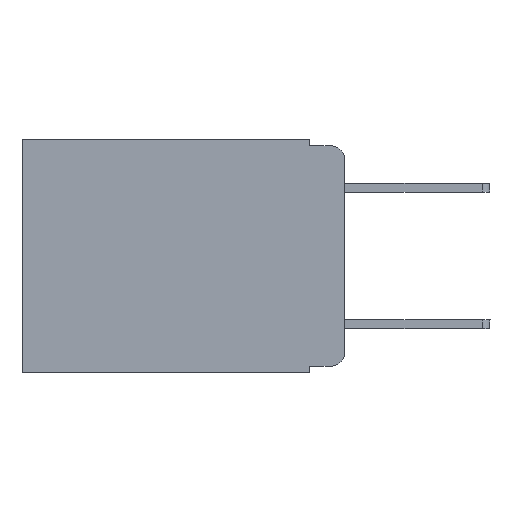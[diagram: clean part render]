
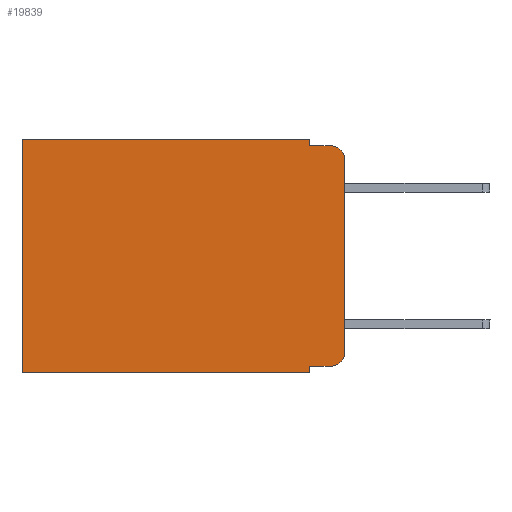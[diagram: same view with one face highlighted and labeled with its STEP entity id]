
A CAD part, left-side view. The second image highlights one B-rep face of the part: STEP entity #19839.
In plain terms, the highlighted planar face has unit normal (-1, 0, 0).
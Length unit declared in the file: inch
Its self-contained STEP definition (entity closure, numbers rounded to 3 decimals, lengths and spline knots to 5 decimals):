
#256 = CARTESIAN_POINT ( 'NONE',  ( 0.298, 0.051, 0. ) ) ;
#275 = VECTOR ( 'NONE', #21660, 39.37008 ) ;
#286 = ORIENTED_EDGE ( 'NONE', *, *, #16755, .T. ) ;
#448 = ORIENTED_EDGE ( 'NONE', *, *, #10956, .F. ) ;
#459 = CARTESIAN_POINT ( 'NONE',  ( 0.298, 0.02, -0.01 ) ) ;
#552 = CARTESIAN_POINT ( 'NONE',  ( 0.298, 0.051, -0.01 ) ) ;
#755 = AXIS2_PLACEMENT_3D ( 'NONE', #16500, #15062, #11660 ) ;
#1377 = EDGE_CURVE ( 'NONE', #11812, #21013, #11252, .T. ) ;
#1898 = FACE_OUTER_BOUND ( 'NONE', #20386, .T. ) ;
#2099 = ORIENTED_EDGE ( 'NONE', *, *, #1377, .F. ) ;
#2185 = LINE ( 'NONE', #2499, #13673 ) ;
#2336 = DIRECTION ( 'NONE',  ( -1., 0., 0. ) ) ;
#2499 = CARTESIAN_POINT ( 'NONE',  ( 0.298, 0.051, 0. ) ) ;
#2699 = CARTESIAN_POINT ( 'NONE',  ( 0.298, 0., 0. ) ) ;
#2823 = DIRECTION ( 'NONE',  ( 0., 1., 0. ) ) ;
#2833 = AXIS2_PLACEMENT_3D ( 'NONE', #18126, #3065, #6771 ) ;
#3065 = DIRECTION ( 'NONE',  ( -1., 0., 0. ) ) ;
#3127 = VERTEX_POINT ( 'NONE', #4134 ) ;
#3799 = VECTOR ( 'NONE', #15537, 39.37008 ) ;
#3920 = EDGE_CURVE ( 'NONE', #7084, #5187, #10862, .T. ) ;
#3995 = CARTESIAN_POINT ( 'NONE',  ( 0.298, 0., -0.313 ) ) ;
#4134 = CARTESIAN_POINT ( 'NONE',  ( 0.298, 0.473, 0. ) ) ;
#4541 = LINE ( 'NONE', #16174, #5563 ) ;
#5187 = VERTEX_POINT ( 'NONE', #459 ) ;
#5304 = CARTESIAN_POINT ( 'NONE',  ( 0.298, 0.02, -0.313 ) ) ;
#5563 = VECTOR ( 'NONE', #21149, 39.37008 ) ;
#5812 = ORIENTED_EDGE ( 'NONE', *, *, #6249, .T. ) ;
#6001 = ORIENTED_EDGE ( 'NONE', *, *, #7471, .F. ) ;
#6236 = VECTOR ( 'NONE', #14060, 39.37008 ) ;
#6249 = EDGE_CURVE ( 'NONE', #7982, #3127, #15973, .T. ) ;
#6476 = CARTESIAN_POINT ( 'NONE',  ( 0.298, 0., -0.343 ) ) ;
#6595 = VERTEX_POINT ( 'NONE', #17065 ) ;
#6627 = CARTESIAN_POINT ( 'NONE',  ( 0.298, 0.02, -0.333 ) ) ;
#6771 = DIRECTION ( 'NONE',  ( 0., 0., -1. ) ) ;
#6863 = ORIENTED_EDGE ( 'NONE', *, *, #15277, .F. ) ;
#7037 = CARTESIAN_POINT ( 'NONE',  ( 0.298, 0.051, -0.01 ) ) ;
#7084 = VERTEX_POINT ( 'NONE', #7037 ) ;
#7381 = DIRECTION ( 'NONE',  ( 0., 0., -1. ) ) ;
#7471 = EDGE_CURVE ( 'NONE', #6595, #19895, #2185, .T. ) ;
#7644 = VECTOR ( 'NONE', #17146, 39.37008 ) ;
#7768 = CARTESIAN_POINT ( 'NONE',  ( 0.298, 0., -0.03 ) ) ;
#7982 = VERTEX_POINT ( 'NONE', #19497 ) ;
#9092 = AXIS2_PLACEMENT_3D ( 'NONE', #5304, #2336, #7381 ) ;
#9336 = LINE ( 'NONE', #14266, #6236 ) ;
#9562 = LINE ( 'NONE', #6476, #275 ) ;
#10462 = LINE ( 'NONE', #256, #3799 ) ;
#10829 = ORIENTED_EDGE ( 'NONE', *, *, #3920, .F. ) ;
#10862 = LINE ( 'NONE', #552, #7644 ) ;
#10956 = EDGE_CURVE ( 'NONE', #7982, #7084, #10462, .T. ) ;
#11252 = LINE ( 'NONE', #2699, #15137 ) ;
#11360 = CARTESIAN_POINT ( 'NONE',  ( 0.298, 0., 0. ) ) ;
#11660 = DIRECTION ( 'NONE',  ( 0., 0., -1. ) ) ;
#11812 = VERTEX_POINT ( 'NONE', #7768 ) ;
#11882 = CIRCLE ( 'NONE', #9092, 0.02 ) ;
#12731 = EDGE_CURVE ( 'NONE', #11812, #5187, #20363, .T. ) ;
#13399 = PLANE ( 'NONE',  #755 ) ;
#13600 = CARTESIAN_POINT ( 'NONE',  ( 0.298, 0.051, -0.343 ) ) ;
#13673 = VECTOR ( 'NONE', #17553, 39.37008 ) ;
#13767 = ORIENTED_EDGE ( 'NONE', *, *, #15201, .T. ) ;
#14060 = DIRECTION ( 'NONE',  ( 0., -1., 0. ) ) ;
#14266 = CARTESIAN_POINT ( 'NONE',  ( 0.298, 0.051, -0.333 ) ) ;
#14274 = CARTESIAN_POINT ( 'NONE',  ( 0.298, 0.473, -0.343 ) ) ;
#14510 = VERTEX_POINT ( 'NONE', #6627 ) ;
#15062 = DIRECTION ( 'NONE',  ( 1., 0., 0. ) ) ;
#15137 = VECTOR ( 'NONE', #21055, 39.37008 ) ;
#15201 = EDGE_CURVE ( 'NONE', #6595, #14510, #9336, .T. ) ;
#15277 = EDGE_CURVE ( 'NONE', #19895, #21073, #9562, .T. ) ;
#15537 = DIRECTION ( 'NONE',  ( 0., 0., -1. ) ) ;
#15842 = EDGE_CURVE ( 'NONE', #3127, #21073, #4541, .T. ) ;
#15973 = LINE ( 'NONE', #11360, #20322 ) ;
#16174 = CARTESIAN_POINT ( 'NONE',  ( 0.298, 0.473, 0. ) ) ;
#16276 = ORIENTED_EDGE ( 'NONE', *, *, #12731, .T. ) ;
#16500 = CARTESIAN_POINT ( 'NONE',  ( 0.298, 0., 0. ) ) ;
#16755 = EDGE_CURVE ( 'NONE', #14510, #21013, #11882, .T. ) ;
#17065 = CARTESIAN_POINT ( 'NONE',  ( 0.298, 0.051, -0.333 ) ) ;
#17146 = DIRECTION ( 'NONE',  ( 0., -1., 0. ) ) ;
#17553 = DIRECTION ( 'NONE',  ( 0., 0., -1. ) ) ;
#18126 = CARTESIAN_POINT ( 'NONE',  ( 0.298, 0.02, -0.03 ) ) ;
#19497 = CARTESIAN_POINT ( 'NONE',  ( 0.298, 0.051, 0. ) ) ;
#19839 = ADVANCED_FACE ( 'NONE', ( #1898 ), #13399, .F. ) ;
#19895 = VERTEX_POINT ( 'NONE', #13600 ) ;
#20322 = VECTOR ( 'NONE', #2823, 39.37008 ) ;
#20363 = CIRCLE ( 'NONE', #2833, 0.02 ) ;
#20386 = EDGE_LOOP ( 'NONE', ( #2099, #16276, #10829, #448, #5812, #20766, #6863, #6001, #13767, #286 ) ) ;
#20766 = ORIENTED_EDGE ( 'NONE', *, *, #15842, .T. ) ;
#21013 = VERTEX_POINT ( 'NONE', #3995 ) ;
#21055 = DIRECTION ( 'NONE',  ( 0., 0., -1. ) ) ;
#21073 = VERTEX_POINT ( 'NONE', #14274 ) ;
#21149 = DIRECTION ( 'NONE',  ( 0., 0., -1. ) ) ;
#21660 = DIRECTION ( 'NONE',  ( 0., 1., 0. ) ) ;
